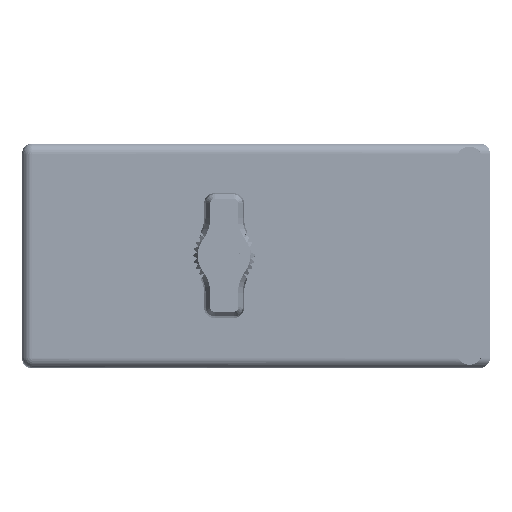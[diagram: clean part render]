
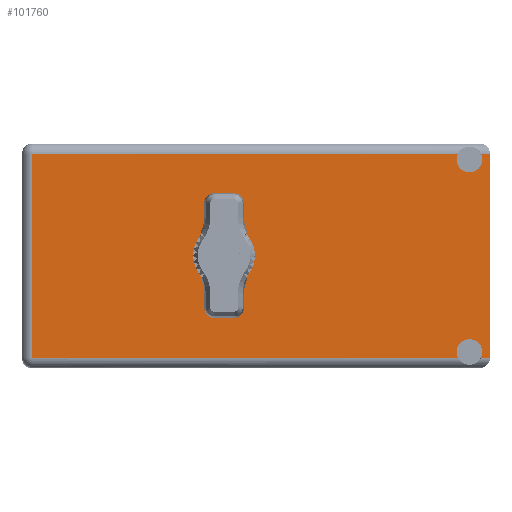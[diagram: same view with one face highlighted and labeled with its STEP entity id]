
A CAD part, top view. The second image highlights one B-rep face of the part: STEP entity #101760.
In plain terms, the highlighted face is planar.
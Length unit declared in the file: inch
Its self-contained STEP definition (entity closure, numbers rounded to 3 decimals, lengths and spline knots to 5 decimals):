
#1291 = CIRCLE ( 'NONE', #80003, 0.17 ) ;
#1786 = VERTEX_POINT ( 'NONE', #109323 ) ;
#6075 = CARTESIAN_POINT ( 'NONE',  ( 3.05, 2.03, -1.421 ) ) ;
#6907 = CARTESIAN_POINT ( 'NONE',  ( 3.19, 2.03, 0. ) ) ;
#7059 = AXIS2_PLACEMENT_3D ( 'NONE', #100311, #117757, #82248 ) ;
#9318 = CARTESIAN_POINT ( 'NONE',  ( 3.19, 2.03, -0.07 ) ) ;
#9487 = ORIENTED_EDGE ( 'NONE', *, *, #113606, .T. ) ;
#11058 = CARTESIAN_POINT ( 'NONE',  ( 1.3775, 2.03, -0.595 ) ) ;
#11565 = CARTESIAN_POINT ( 'NONE',  ( 3.19, 2.03, -0.07 ) ) ;
#11889 = EDGE_CURVE ( 'NONE', #71498, #86187, #89324, .T. ) ;
#12118 = AXIS2_PLACEMENT_3D ( 'NONE', #15897, #78525, #32207 ) ;
#12523 = EDGE_CURVE ( 'NONE', #104494, #107676, #76342, .T. ) ;
#12802 = CARTESIAN_POINT ( 'NONE',  ( 3.05, 2.03, -1.421 ) ) ;
#13002 = DIRECTION ( 'NONE',  ( 0., 1., 0. ) ) ;
#15897 = CARTESIAN_POINT ( 'NONE',  ( 3.05, 2.03, -0.109 ) ) ;
#16341 = VERTEX_POINT ( 'NONE', #59568 ) ;
#18028 = FACE_BOUND ( 'NONE', #106971, .T. ) ;
#18674 = CARTESIAN_POINT ( 'NONE',  ( 3.05, 2.03, -1.3335 ) ) ;
#19125 = CARTESIAN_POINT ( 'NONE',  ( 1.3775, 2.03, -0.765 ) ) ;
#19142 = AXIS2_PLACEMENT_3D ( 'NONE', #95448, #13002, #52007 ) ;
#19516 = AXIS2_PLACEMENT_3D ( 'NONE', #6075, #113837, #59070 ) ;
#20884 = CARTESIAN_POINT ( 'NONE',  ( 0., 2.03, -1.46 ) ) ;
#20886 = DIRECTION ( 'NONE',  ( -1., 0., 0. ) ) ;
#21109 = VERTEX_POINT ( 'NONE', #94947 ) ;
#21709 = VERTEX_POINT ( 'NONE', #103106 ) ;
#22885 = ORIENTED_EDGE ( 'NONE', *, *, #11889, .F. ) ;
#24142 = CARTESIAN_POINT ( 'NONE',  ( 3.19, 2.03, -1.46 ) ) ;
#25113 = LINE ( 'NONE', #100337, #68952 ) ;
#25745 = DIRECTION ( 'NONE',  ( 0., 1., 0. ) ) ;
#28763 = CIRCLE ( 'NONE', #19142, 0.0875 ) ;
#30415 = VECTOR ( 'NONE', #20886, 39.37008 ) ;
#31416 = DIRECTION ( 'NONE',  ( 0., 1., 0. ) ) ;
#32207 = DIRECTION ( 'NONE',  ( 0., 0., 1. ) ) ;
#36281 = CARTESIAN_POINT ( 'NONE',  ( 0.07, 2.03, -1.46 ) ) ;
#36311 = ORIENTED_EDGE ( 'NONE', *, *, #111256, .F. ) ;
#37630 = ORIENTED_EDGE ( 'NONE', *, *, #117135, .F. ) ;
#39077 = DIRECTION ( 'NONE',  ( 0., 0., 1. ) ) ;
#43589 = DIRECTION ( 'NONE',  ( 0., 0., 1. ) ) ;
#43948 = ORIENTED_EDGE ( 'NONE', *, *, #98431, .T. ) ;
#46750 = LINE ( 'NONE', #102746, #30415 ) ;
#47263 = ORIENTED_EDGE ( 'NONE', *, *, #49172, .T. ) ;
#47665 = ORIENTED_EDGE ( 'NONE', *, *, #65379, .F. ) ;
#48089 = DIRECTION ( 'NONE',  ( 0., 1., 0. ) ) ;
#48107 = ORIENTED_EDGE ( 'NONE', *, *, #12523, .T. ) ;
#49172 = EDGE_CURVE ( 'NONE', #71498, #21709, #46750, .T. ) ;
#52007 = DIRECTION ( 'NONE',  ( 0., 0., 1. ) ) ;
#58171 = DIRECTION ( 'NONE',  ( -1., 0., 0. ) ) ;
#58507 = CARTESIAN_POINT ( 'NONE',  ( 0.07, 2.03, -0.07 ) ) ;
#59070 = DIRECTION ( 'NONE',  ( 0., 0., 1. ) ) ;
#59568 = CARTESIAN_POINT ( 'NONE',  ( 2.97167, 2.03, -0.07 ) ) ;
#60234 = LINE ( 'NONE', #11565, #111185 ) ;
#62094 = EDGE_CURVE ( 'NONE', #118654, #21109, #1291, .T. ) ;
#65379 = EDGE_CURVE ( 'NONE', #98533, #1786, #90849, .T. ) ;
#67590 = ORIENTED_EDGE ( 'NONE', *, *, #88338, .F. ) ;
#68952 = VECTOR ( 'NONE', #90695, 39.37008 ) ;
#69105 = VECTOR ( 'NONE', #58171, 39.37008 ) ;
#69728 = VECTOR ( 'NONE', #84773, 39.37008 ) ;
#70673 = ORIENTED_EDGE ( 'NONE', *, *, #62094, .F. ) ;
#71498 = VERTEX_POINT ( 'NONE', #24142 ) ;
#72635 = CARTESIAN_POINT ( 'NONE',  ( 2.97167, 2.03, -1.46 ) ) ;
#73710 = AXIS2_PLACEMENT_3D ( 'NONE', #12802, #31416, #112709 ) ;
#74257 = VERTEX_POINT ( 'NONE', #18674 ) ;
#75891 = CIRCLE ( 'NONE', #73710, 0.0875 ) ;
#76342 = LINE ( 'NONE', #82542, #69728 ) ;
#78525 = DIRECTION ( 'NONE',  ( 0., 1., 0. ) ) ;
#80003 = AXIS2_PLACEMENT_3D ( 'NONE', #19125, #25745, #92544 ) ;
#81557 = ORIENTED_EDGE ( 'NONE', *, *, #84247, .T. ) ;
#82248 = DIRECTION ( 'NONE',  ( 0., 0., 1. ) ) ;
#82542 = CARTESIAN_POINT ( 'NONE',  ( 0.07, 2.03, -1.53 ) ) ;
#83133 = VECTOR ( 'NONE', #43589, 39.37008 ) ;
#84247 = EDGE_CURVE ( 'NONE', #87136, #104494, #103343, .T. ) ;
#84393 = ORIENTED_EDGE ( 'NONE', *, *, #107655, .F. ) ;
#84773 = DIRECTION ( 'NONE',  ( 0., 0., 1. ) ) ;
#84902 = CIRCLE ( 'NONE', #19516, 0.0875 ) ;
#84953 = DIRECTION ( 'NONE',  ( 1., 0., 0. ) ) ;
#86187 = VERTEX_POINT ( 'NONE', #9318 ) ;
#87136 = VERTEX_POINT ( 'NONE', #72635 ) ;
#88338 = EDGE_CURVE ( 'NONE', #74257, #21709, #84902, .T. ) ;
#89324 = LINE ( 'NONE', #6907, #83133 ) ;
#90695 = DIRECTION ( 'NONE',  ( 1., 0., 0. ) ) ;
#90849 = CIRCLE ( 'NONE', #12118, 0.0875 ) ;
#92505 = CARTESIAN_POINT ( 'NONE',  ( 3.12833, 2.03, -0.07 ) ) ;
#92544 = DIRECTION ( 'NONE',  ( 0., 0., 1. ) ) ;
#93866 = FACE_OUTER_BOUND ( 'NONE', #107823, .T. ) ;
#94947 = CARTESIAN_POINT ( 'NONE',  ( 1.3775, 2.03, -0.935 ) ) ;
#95448 = CARTESIAN_POINT ( 'NONE',  ( 3.05, 2.03, -0.109 ) ) ;
#96549 = AXIS2_PLACEMENT_3D ( 'NONE', #111326, #48089, #39077 ) ;
#98431 = EDGE_CURVE ( 'NONE', #98533, #86187, #25113, .T. ) ;
#98533 = VERTEX_POINT ( 'NONE', #92505 ) ;
#100311 = CARTESIAN_POINT ( 'NONE',  ( 1.3775, 2.03, -0.765 ) ) ;
#100337 = CARTESIAN_POINT ( 'NONE',  ( 3.19, 2.03, -0.07 ) ) ;
#101760 = ADVANCED_FACE ( 'NONE', ( #18028, #93866 ), #102299, .T. ) ;
#102299 = PLANE ( 'NONE',  #96549 ) ;
#102746 = CARTESIAN_POINT ( 'NONE',  ( 0., 2.03, -1.46 ) ) ;
#103106 = CARTESIAN_POINT ( 'NONE',  ( 3.12833, 2.03, -1.46 ) ) ;
#103343 = LINE ( 'NONE', #20884, #69105 ) ;
#104494 = VERTEX_POINT ( 'NONE', #36281 ) ;
#106971 = EDGE_LOOP ( 'NONE', ( #70673, #36311 ) ) ;
#107655 = EDGE_CURVE ( 'NONE', #87136, #74257, #75891, .T. ) ;
#107676 = VERTEX_POINT ( 'NONE', #58507 ) ;
#107823 = EDGE_LOOP ( 'NONE', ( #9487, #37630, #47665, #43948, #22885, #47263, #67590, #84393, #81557, #48107 ) ) ;
#109323 = CARTESIAN_POINT ( 'NONE',  ( 3.05, 2.03, -0.1965 ) ) ;
#111185 = VECTOR ( 'NONE', #84953, 39.37008 ) ;
#111256 = EDGE_CURVE ( 'NONE', #21109, #118654, #118473, .T. ) ;
#111326 = CARTESIAN_POINT ( 'NONE',  ( 0., 2.03, -1.53 ) ) ;
#112709 = DIRECTION ( 'NONE',  ( 0., 0., 1. ) ) ;
#113606 = EDGE_CURVE ( 'NONE', #107676, #16341, #60234, .T. ) ;
#113837 = DIRECTION ( 'NONE',  ( 0., 1., 0. ) ) ;
#117135 = EDGE_CURVE ( 'NONE', #1786, #16341, #28763, .T. ) ;
#117757 = DIRECTION ( 'NONE',  ( 0., 1., 0. ) ) ;
#118473 = CIRCLE ( 'NONE', #7059, 0.17 ) ;
#118654 = VERTEX_POINT ( 'NONE', #11058 ) ;
